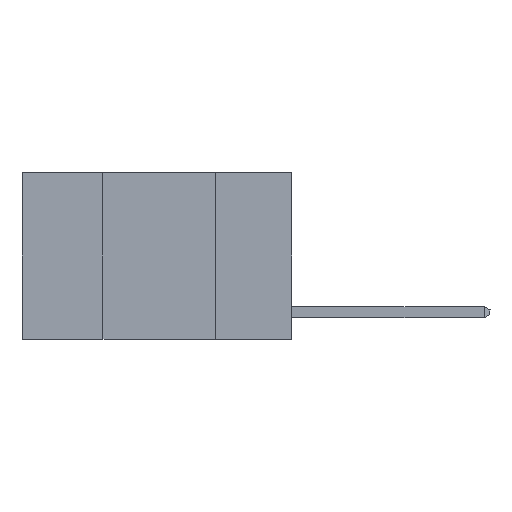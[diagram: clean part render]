
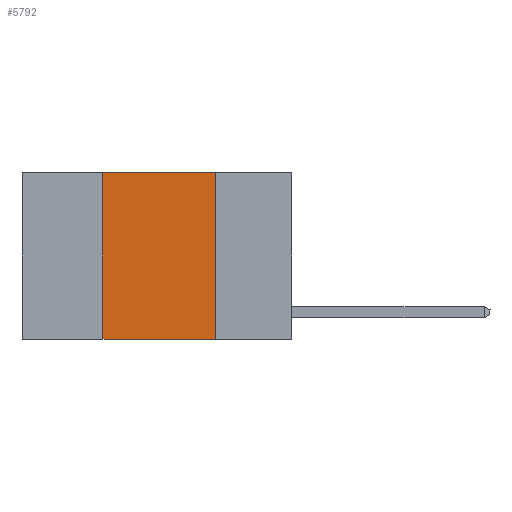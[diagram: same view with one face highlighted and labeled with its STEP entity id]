
A CAD part, left-side view. The second image highlights one B-rep face of the part: STEP entity #5792.
In plain terms, the highlighted planar face has unit normal (-1, 0, 0).
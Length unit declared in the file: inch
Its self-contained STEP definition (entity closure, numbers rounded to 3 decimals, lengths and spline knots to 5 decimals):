
#33 = LINE ( 'NONE', #6218, #17347 ) ;
#579 = EDGE_CURVE ( 'NONE', #16062, #6496, #16227, .T. ) ;
#1041 = EDGE_CURVE ( 'NONE', #11792, #16062, #5628, .T. ) ;
#1212 = CARTESIAN_POINT ( 'NONE',  ( 0., 0.42, 0. ) ) ;
#1444 = DIRECTION ( 'NONE',  ( 0., 0., -1. ) ) ;
#2497 = CARTESIAN_POINT ( 'NONE',  ( 0., 0.17, 0. ) ) ;
#3157 = EDGE_CURVE ( 'NONE', #6496, #3996, #5483, .T. ) ;
#3452 = DIRECTION ( 'NONE',  ( 0., -1., 0. ) ) ;
#3456 = ORIENTED_EDGE ( 'NONE', *, *, #3157, .F. ) ;
#3830 = DIRECTION ( 'NONE',  ( 0., 0., -1. ) ) ;
#3996 = VERTEX_POINT ( 'NONE', #17756 ) ;
#4021 = VECTOR ( 'NONE', #9440, 39.37008 ) ;
#5451 = ORIENTED_EDGE ( 'NONE', *, *, #1041, .F. ) ;
#5483 = LINE ( 'NONE', #12186, #9132 ) ;
#5504 = DIRECTION ( 'NONE',  ( 1., 0., 0. ) ) ;
#5628 = LINE ( 'NONE', #1212, #9018 ) ;
#5792 = ADVANCED_FACE ( 'NONE', ( #7062 ), #14124, .F. ) ;
#6218 = CARTESIAN_POINT ( 'NONE',  ( 0., 0.6, -0.37 ) ) ;
#6496 = VERTEX_POINT ( 'NONE', #2497 ) ;
#7062 = FACE_OUTER_BOUND ( 'NONE', #17686, .T. ) ;
#7300 = ORIENTED_EDGE ( 'NONE', *, *, #14115, .T. ) ;
#8281 = ORIENTED_EDGE ( 'NONE', *, *, #579, .F. ) ;
#8970 = AXIS2_PLACEMENT_3D ( 'NONE', #16811, #5504, #1444 ) ;
#9018 = VECTOR ( 'NONE', #18116, 39.37008 ) ;
#9132 = VECTOR ( 'NONE', #3830, 39.37008 ) ;
#9440 = DIRECTION ( 'NONE',  ( 0., -1., 0. ) ) ;
#11792 = VERTEX_POINT ( 'NONE', #12411 ) ;
#12186 = CARTESIAN_POINT ( 'NONE',  ( 0., 0.17, 0. ) ) ;
#12411 = CARTESIAN_POINT ( 'NONE',  ( 0., 0.42, -0.37 ) ) ;
#14115 = EDGE_CURVE ( 'NONE', #11792, #3996, #33, .T. ) ;
#14124 = PLANE ( 'NONE',  #8970 ) ;
#14944 = CARTESIAN_POINT ( 'NONE',  ( 0., 0.6, 0. ) ) ;
#16062 = VERTEX_POINT ( 'NONE', #17591 ) ;
#16227 = LINE ( 'NONE', #14944, #4021 ) ;
#16811 = CARTESIAN_POINT ( 'NONE',  ( 0., 0.6, 0. ) ) ;
#17347 = VECTOR ( 'NONE', #3452, 39.37008 ) ;
#17591 = CARTESIAN_POINT ( 'NONE',  ( 0., 0.42, 0. ) ) ;
#17686 = EDGE_LOOP ( 'NONE', ( #3456, #8281, #5451, #7300 ) ) ;
#17756 = CARTESIAN_POINT ( 'NONE',  ( 0., 0.17, -0.37 ) ) ;
#18116 = DIRECTION ( 'NONE',  ( 0., 0., 1. ) ) ;
